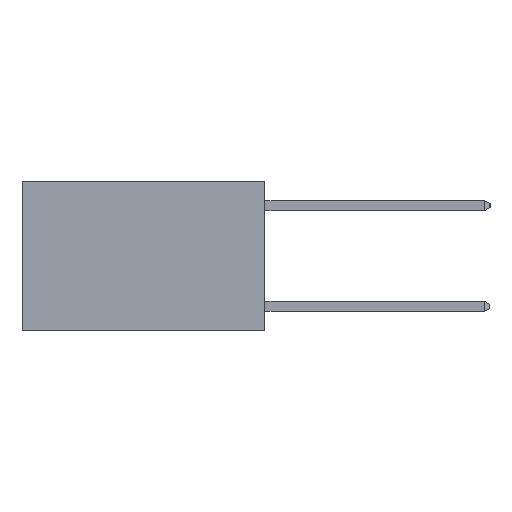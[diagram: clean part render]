
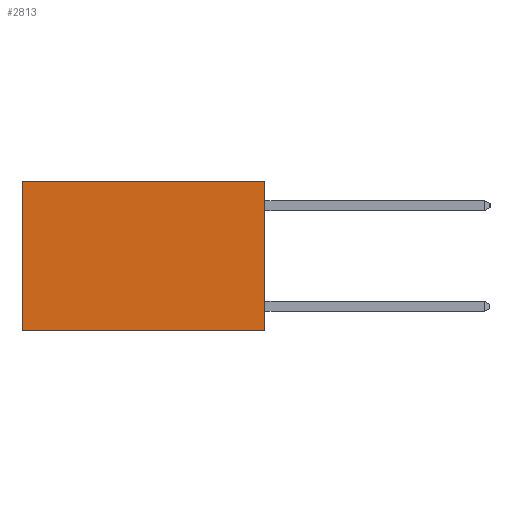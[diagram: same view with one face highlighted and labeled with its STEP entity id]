
A CAD part, left-side view. The second image highlights one B-rep face of the part: STEP entity #2813.
In plain terms, the highlighted planar face has unit normal (-1, 0, 0).
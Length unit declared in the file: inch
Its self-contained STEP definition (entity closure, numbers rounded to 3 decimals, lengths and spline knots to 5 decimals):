
#178 = LINE ( 'NONE', #4597, #1919 ) ;
#867 = LINE ( 'NONE', #3258, #5718 ) ;
#951 = DIRECTION ( 'NONE',  ( 0., 1., 0. ) ) ;
#1120 = DIRECTION ( 'NONE',  ( 0., 0., -1. ) ) ;
#1302 = EDGE_CURVE ( 'NONE', #2883, #6761, #178, .T. ) ;
#1321 = VERTEX_POINT ( 'NONE', #4009 ) ;
#1689 = EDGE_CURVE ( 'NONE', #2883, #1321, #867, .T. ) ;
#1871 = ORIENTED_EDGE ( 'NONE', *, *, #1689, .F. ) ;
#1919 = VECTOR ( 'NONE', #2694, 39.37008 ) ;
#1993 = EDGE_LOOP ( 'NONE', ( #3772, #5847, #1871, #6498 ) ) ;
#2105 = VECTOR ( 'NONE', #3844, 39.37008 ) ;
#2277 = CARTESIAN_POINT ( 'NONE',  ( 0.2625, 0., -0.37 ) ) ;
#2369 = EDGE_CURVE ( 'NONE', #6761, #7453, #4289, .T. ) ;
#2694 = DIRECTION ( 'NONE',  ( 0., 1., 0. ) ) ;
#2813 = ADVANCED_FACE ( 'NONE', ( #5706 ), #7893, .F. ) ;
#2883 = VERTEX_POINT ( 'NONE', #3810 ) ;
#3242 = CARTESIAN_POINT ( 'NONE',  ( 0.2625, 0.6, -0.37 ) ) ;
#3258 = CARTESIAN_POINT ( 'NONE',  ( 0.2625, 0., 0. ) ) ;
#3488 = EDGE_CURVE ( 'NONE', #1321, #7453, #6525, .T. ) ;
#3772 = ORIENTED_EDGE ( 'NONE', *, *, #2369, .T. ) ;
#3810 = CARTESIAN_POINT ( 'NONE',  ( 0.2625, 0., 0. ) ) ;
#3844 = DIRECTION ( 'NONE',  ( 0., 0., -1. ) ) ;
#4009 = CARTESIAN_POINT ( 'NONE',  ( 0.2625, 0., -0.37 ) ) ;
#4289 = LINE ( 'NONE', #5664, #2105 ) ;
#4359 = CARTESIAN_POINT ( 'NONE',  ( 0.2625, 0., 0. ) ) ;
#4597 = CARTESIAN_POINT ( 'NONE',  ( 0.2625, 0., 0. ) ) ;
#4882 = AXIS2_PLACEMENT_3D ( 'NONE', #4359, #4964, #1120 ) ;
#4964 = DIRECTION ( 'NONE',  ( 1., 0., 0. ) ) ;
#5149 = DIRECTION ( 'NONE',  ( 0., 0., -1. ) ) ;
#5664 = CARTESIAN_POINT ( 'NONE',  ( 0.2625, 0.6, 0. ) ) ;
#5706 = FACE_OUTER_BOUND ( 'NONE', #1993, .T. ) ;
#5718 = VECTOR ( 'NONE', #5149, 39.37008 ) ;
#5847 = ORIENTED_EDGE ( 'NONE', *, *, #3488, .F. ) ;
#6498 = ORIENTED_EDGE ( 'NONE', *, *, #1302, .T. ) ;
#6525 = LINE ( 'NONE', #2277, #6707 ) ;
#6707 = VECTOR ( 'NONE', #951, 39.37008 ) ;
#6761 = VERTEX_POINT ( 'NONE', #7613 ) ;
#7453 = VERTEX_POINT ( 'NONE', #3242 ) ;
#7613 = CARTESIAN_POINT ( 'NONE',  ( 0.2625, 0.6, 0. ) ) ;
#7893 = PLANE ( 'NONE',  #4882 ) ;
